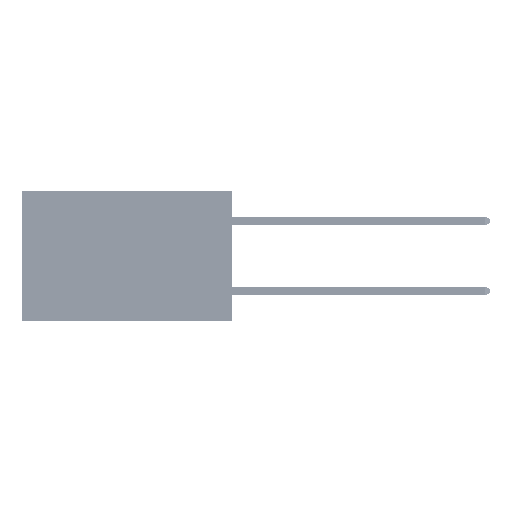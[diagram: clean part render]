
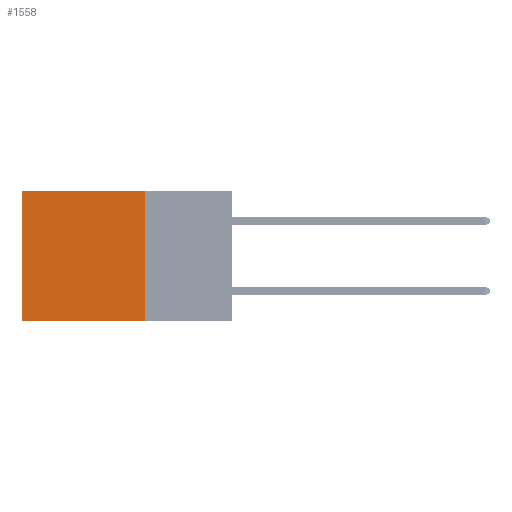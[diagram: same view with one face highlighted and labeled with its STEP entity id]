
A CAD part, left-side view. The second image highlights one B-rep face of the part: STEP entity #1558.
In plain terms, the highlighted planar face has unit normal (-1, 0, 0).
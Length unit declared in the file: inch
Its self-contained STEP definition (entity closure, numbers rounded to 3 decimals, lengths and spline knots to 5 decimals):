
#72 = AXIS2_PLACEMENT_3D ( 'NONE', #34389, #13016, #9710 ) ;
#482 = VERTEX_POINT ( 'NONE', #38827 ) ;
#1558 = ADVANCED_FACE ( 'NONE', ( #20064 ), #41901, .F. ) ;
#2313 = EDGE_CURVE ( 'NONE', #23714, #16558, #34379, .T. ) ;
#6102 = CARTESIAN_POINT ( 'NONE',  ( 0.2875, 0.6, 0. ) ) ;
#6663 = CARTESIAN_POINT ( 'NONE',  ( 0.2875, 0.25, -0.37 ) ) ;
#7909 = CARTESIAN_POINT ( 'NONE',  ( 0.2875, 0.6, -0.37 ) ) ;
#9710 = DIRECTION ( 'NONE',  ( 0., 0., -1. ) ) ;
#13016 = DIRECTION ( 'NONE',  ( 1., 0., 0. ) ) ;
#13507 = EDGE_LOOP ( 'NONE', ( #33893, #24369, #35958, #45226 ) ) ;
#15303 = VECTOR ( 'NONE', #39339, 39.37008 ) ;
#16558 = VERTEX_POINT ( 'NONE', #29511 ) ;
#16694 = VECTOR ( 'NONE', #17388, 39.37008 ) ;
#17388 = DIRECTION ( 'NONE',  ( 0., 0., -1. ) ) ;
#20064 = FACE_OUTER_BOUND ( 'NONE', #13507, .T. ) ;
#20424 = VERTEX_POINT ( 'NONE', #7909 ) ;
#20653 = EDGE_CURVE ( 'NONE', #16558, #20424, #32288, .T. ) ;
#21137 = LINE ( 'NONE', #6102, #16694 ) ;
#23607 = VECTOR ( 'NONE', #45430, 39.37008 ) ;
#23714 = VERTEX_POINT ( 'NONE', #39459 ) ;
#24369 = ORIENTED_EDGE ( 'NONE', *, *, #20653, .F. ) ;
#25012 = CARTESIAN_POINT ( 'NONE',  ( 0.2875, 0.25, 0. ) ) ;
#28322 = LINE ( 'NONE', #25012, #30423 ) ;
#29511 = CARTESIAN_POINT ( 'NONE',  ( 0.2875, 0.25, -0.37 ) ) ;
#30423 = VECTOR ( 'NONE', #39354, 39.37008 ) ;
#31995 = EDGE_CURVE ( 'NONE', #482, #20424, #21137, .T. ) ;
#32288 = LINE ( 'NONE', #6663, #15303 ) ;
#33893 = ORIENTED_EDGE ( 'NONE', *, *, #31995, .T. ) ;
#34379 = LINE ( 'NONE', #37680, #23607 ) ;
#34389 = CARTESIAN_POINT ( 'NONE',  ( 0.2875, 0.25, 0. ) ) ;
#35958 = ORIENTED_EDGE ( 'NONE', *, *, #2313, .F. ) ;
#37680 = CARTESIAN_POINT ( 'NONE',  ( 0.2875, 0.25, 0. ) ) ;
#38827 = CARTESIAN_POINT ( 'NONE',  ( 0.2875, 0.6, 0. ) ) ;
#39339 = DIRECTION ( 'NONE',  ( 0., 1., 0. ) ) ;
#39354 = DIRECTION ( 'NONE',  ( 0., 1., 0. ) ) ;
#39459 = CARTESIAN_POINT ( 'NONE',  ( 0.2875, 0.25, 0. ) ) ;
#41901 = PLANE ( 'NONE',  #72 ) ;
#42422 = EDGE_CURVE ( 'NONE', #23714, #482, #28322, .T. ) ;
#45226 = ORIENTED_EDGE ( 'NONE', *, *, #42422, .T. ) ;
#45430 = DIRECTION ( 'NONE',  ( 0., 0., -1. ) ) ;
